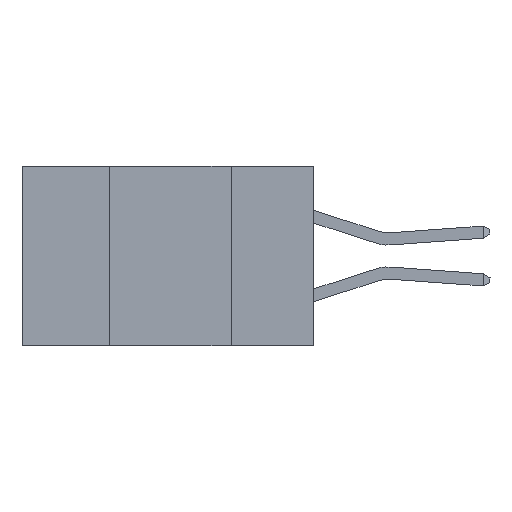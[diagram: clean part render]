
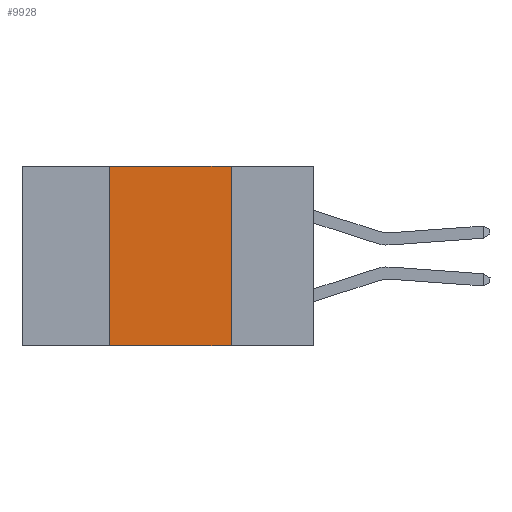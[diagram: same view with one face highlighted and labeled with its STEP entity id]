
A CAD part, left-side view. The second image highlights one B-rep face of the part: STEP entity #9928.
In plain terms, the highlighted planar face has unit normal (-1, 0, 0).
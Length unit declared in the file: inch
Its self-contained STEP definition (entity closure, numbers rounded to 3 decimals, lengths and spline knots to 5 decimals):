
#533 = EDGE_CURVE ( 'NONE', #3707, #6416, #21009, .T. ) ;
#1518 = DIRECTION ( 'NONE',  ( 0., 0., -1. ) ) ;
#1763 = CARTESIAN_POINT ( 'NONE',  ( 0., 0.42, 0. ) ) ;
#1831 = DIRECTION ( 'NONE',  ( 0., 0., -1. ) ) ;
#2679 = CARTESIAN_POINT ( 'NONE',  ( 0., 0.6, 0. ) ) ;
#2903 = VECTOR ( 'NONE', #1518, 39.37008 ) ;
#2979 = LINE ( 'NONE', #9408, #21697 ) ;
#3682 = CARTESIAN_POINT ( 'NONE',  ( 0., 0.17, -0.37 ) ) ;
#3707 = VERTEX_POINT ( 'NONE', #6662 ) ;
#4643 = DIRECTION ( 'NONE',  ( 0., -1., 0. ) ) ;
#4960 = VECTOR ( 'NONE', #4643, 39.37008 ) ;
#5716 = EDGE_LOOP ( 'NONE', ( #23970, #21127, #6346, #24705 ) ) ;
#6346 = ORIENTED_EDGE ( 'NONE', *, *, #25011, .F. ) ;
#6416 = VERTEX_POINT ( 'NONE', #3682 ) ;
#6662 = CARTESIAN_POINT ( 'NONE',  ( 0., 0.17, 0. ) ) ;
#8520 = VERTEX_POINT ( 'NONE', #24019 ) ;
#9408 = CARTESIAN_POINT ( 'NONE',  ( 0., 0.6, -0.37 ) ) ;
#9928 = ADVANCED_FACE ( 'NONE', ( #21755 ), #21236, .F. ) ;
#10562 = EDGE_CURVE ( 'NONE', #14228, #3707, #14497, .T. ) ;
#11327 = CARTESIAN_POINT ( 'NONE',  ( 0., 0.6, 0. ) ) ;
#11407 = DIRECTION ( 'NONE',  ( 1., 0., 0. ) ) ;
#13296 = CARTESIAN_POINT ( 'NONE',  ( 0., 0.42, 0. ) ) ;
#14228 = VERTEX_POINT ( 'NONE', #13296 ) ;
#14497 = LINE ( 'NONE', #2679, #4960 ) ;
#16175 = AXIS2_PLACEMENT_3D ( 'NONE', #11327, #11407, #1831 ) ;
#17168 = CARTESIAN_POINT ( 'NONE',  ( 0., 0.17, 0. ) ) ;
#17304 = LINE ( 'NONE', #1763, #17597 ) ;
#17597 = VECTOR ( 'NONE', #17664, 39.37008 ) ;
#17664 = DIRECTION ( 'NONE',  ( 0., 0., 1. ) ) ;
#21009 = LINE ( 'NONE', #17168, #2903 ) ;
#21127 = ORIENTED_EDGE ( 'NONE', *, *, #10562, .F. ) ;
#21236 = PLANE ( 'NONE',  #16175 ) ;
#21697 = VECTOR ( 'NONE', #25184, 39.37008 ) ;
#21755 = FACE_OUTER_BOUND ( 'NONE', #5716, .T. ) ;
#21924 = EDGE_CURVE ( 'NONE', #8520, #6416, #2979, .T. ) ;
#23970 = ORIENTED_EDGE ( 'NONE', *, *, #533, .F. ) ;
#24019 = CARTESIAN_POINT ( 'NONE',  ( 0., 0.42, -0.37 ) ) ;
#24705 = ORIENTED_EDGE ( 'NONE', *, *, #21924, .T. ) ;
#25011 = EDGE_CURVE ( 'NONE', #8520, #14228, #17304, .T. ) ;
#25184 = DIRECTION ( 'NONE',  ( 0., -1., 0. ) ) ;
